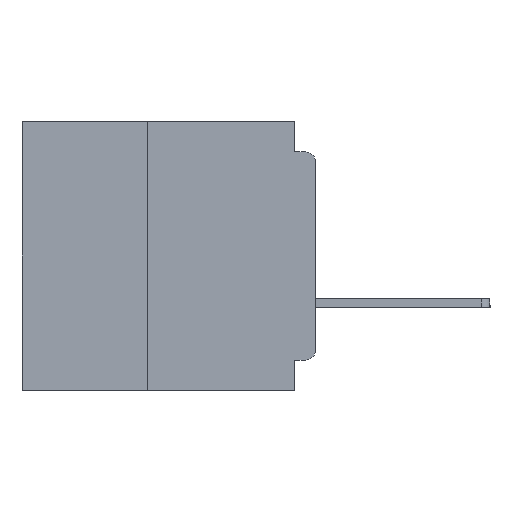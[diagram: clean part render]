
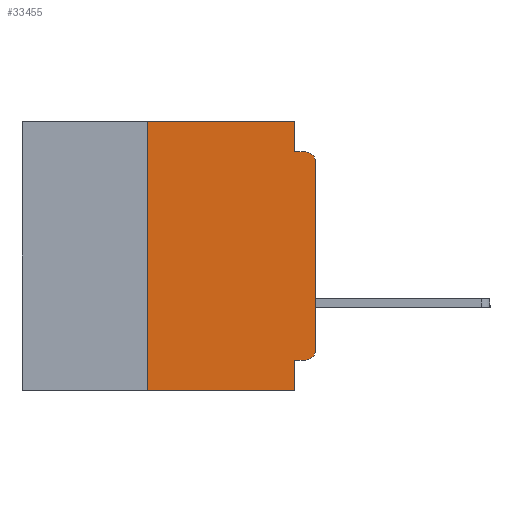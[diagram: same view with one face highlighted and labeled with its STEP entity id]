
A CAD part, left-side view. The second image highlights one B-rep face of the part: STEP entity #33455.
In plain terms, the highlighted planar face has unit normal (-1, 0, 0).
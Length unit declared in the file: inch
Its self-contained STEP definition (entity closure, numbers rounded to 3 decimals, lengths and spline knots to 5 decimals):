
#30 = LINE ( 'NONE', #48279, #38272 ) ;
#171 = EDGE_CURVE ( 'NONE', #45101, #15262, #49814, .T. ) ;
#313 = ORIENTED_EDGE ( 'NONE', *, *, #45970, .F. ) ;
#551 = EDGE_CURVE ( 'NONE', #40416, #3719, #44306, .T. ) ;
#1659 = VECTOR ( 'NONE', #46915, 39.37008 ) ;
#2421 = CARTESIAN_POINT ( 'NONE',  ( 0., 0.031, 0. ) ) ;
#3719 = VERTEX_POINT ( 'NONE', #20917 ) ;
#3792 = LINE ( 'NONE', #22069, #23564 ) ;
#4035 = ORIENTED_EDGE ( 'NONE', *, *, #551, .F. ) ;
#8133 = EDGE_CURVE ( 'NONE', #45101, #36165, #47011, .T. ) ;
#9137 = DIRECTION ( 'NONE',  ( 0., 0., -1. ) ) ;
#9287 = DIRECTION ( 'NONE',  ( 0., 0., 1. ) ) ;
#9511 = DIRECTION ( 'NONE',  ( 0., 0., 1. ) ) ;
#9657 = CARTESIAN_POINT ( 'NONE',  ( 0., 0.015, -0.34 ) ) ;
#10088 = VERTEX_POINT ( 'NONE', #45412 ) ;
#10184 = ORIENTED_EDGE ( 'NONE', *, *, #13428, .F. ) ;
#11434 = AXIS2_PLACEMENT_3D ( 'NONE', #20685, #48061, #24645 ) ;
#12172 = LINE ( 'NONE', #31227, #1659 ) ;
#12761 = LINE ( 'NONE', #40751, #50782 ) ;
#12777 = FACE_OUTER_BOUND ( 'NONE', #46344, .T. ) ;
#12969 = VECTOR ( 'NONE', #26232, 39.37008 ) ;
#13257 = ORIENTED_EDGE ( 'NONE', *, *, #41112, .T. ) ;
#13428 = EDGE_CURVE ( 'NONE', #44239, #15635, #27685, .T. ) ;
#13634 = DIRECTION ( 'NONE',  ( 0., 0., -1. ) ) ;
#14319 = CARTESIAN_POINT ( 'NONE',  ( 0., 0.25, 0. ) ) ;
#15262 = VERTEX_POINT ( 'NONE', #15535 ) ;
#15535 = CARTESIAN_POINT ( 'NONE',  ( 0., 0.031, -0.4 ) ) ;
#15635 = VERTEX_POINT ( 'NONE', #22401 ) ;
#15716 = VECTOR ( 'NONE', #9511, 39.37008 ) ;
#15987 = VECTOR ( 'NONE', #24938, 39.37008 ) ;
#16967 = ORIENTED_EDGE ( 'NONE', *, *, #19109, .F. ) ;
#17752 = DIRECTION ( 'NONE',  ( 0., -1., 0. ) ) ;
#18827 = CARTESIAN_POINT ( 'NONE',  ( 0., 0., -0.34 ) ) ;
#19109 = EDGE_CURVE ( 'NONE', #15635, #42695, #3792, .T. ) ;
#19437 = CARTESIAN_POINT ( 'NONE',  ( 0., 0.25, -0.4 ) ) ;
#19502 = CARTESIAN_POINT ( 'NONE',  ( 0., 0.437, 0. ) ) ;
#19772 = CIRCLE ( 'NONE', #11434, 0.015 ) ;
#20685 = CARTESIAN_POINT ( 'NONE',  ( 0., 0.015, -0.06 ) ) ;
#20917 = CARTESIAN_POINT ( 'NONE',  ( 0., 0.031, -0.355 ) ) ;
#20986 = CARTESIAN_POINT ( 'NONE',  ( 0., 0.031, 0. ) ) ;
#20989 = CARTESIAN_POINT ( 'NONE',  ( 0., 0.437, -0.4 ) ) ;
#22069 = CARTESIAN_POINT ( 'NONE',  ( 0., 0., -0.045 ) ) ;
#22242 = DIRECTION ( 'NONE',  ( 0., -1., 0. ) ) ;
#22401 = CARTESIAN_POINT ( 'NONE',  ( 0., 0.031, -0.045 ) ) ;
#22969 = CARTESIAN_POINT ( 'NONE',  ( 0., 0., -0.355 ) ) ;
#23477 = DIRECTION ( 'NONE',  ( 0., 0., -1. ) ) ;
#23564 = VECTOR ( 'NONE', #22242, 39.37008 ) ;
#24240 = CIRCLE ( 'NONE', #46910, 0.015 ) ;
#24417 = ORIENTED_EDGE ( 'NONE', *, *, #8133, .F. ) ;
#24645 = DIRECTION ( 'NONE',  ( 0., 0., -1. ) ) ;
#24938 = DIRECTION ( 'NONE',  ( 0., 0., -1. ) ) ;
#26232 = DIRECTION ( 'NONE',  ( 0., 1., 0. ) ) ;
#27685 = LINE ( 'NONE', #20986, #15987 ) ;
#28710 = ORIENTED_EDGE ( 'NONE', *, *, #30641, .T. ) ;
#29152 = CARTESIAN_POINT ( 'NONE',  ( 0., 0.25, -0.4 ) ) ;
#30289 = VECTOR ( 'NONE', #17752, 39.37008 ) ;
#30641 = EDGE_CURVE ( 'NONE', #40416, #44302, #24240, .T. ) ;
#31167 = ORIENTED_EDGE ( 'NONE', *, *, #42493, .F. ) ;
#31227 = CARTESIAN_POINT ( 'NONE',  ( 0., 0.437, 0. ) ) ;
#33455 = ADVANCED_FACE ( 'NONE', ( #12777 ), #42973, .F. ) ;
#35858 = CARTESIAN_POINT ( 'NONE',  ( 0., 0.015, -0.355 ) ) ;
#36165 = VERTEX_POINT ( 'NONE', #14319 ) ;
#37200 = DIRECTION ( 'NONE',  ( -1., 0., 0. ) ) ;
#38272 = VECTOR ( 'NONE', #9137, 39.37008 ) ;
#39702 = ORIENTED_EDGE ( 'NONE', *, *, #42759, .T. ) ;
#40416 = VERTEX_POINT ( 'NONE', #35858 ) ;
#40751 = CARTESIAN_POINT ( 'NONE',  ( 0., 0., 0. ) ) ;
#41112 = EDGE_CURVE ( 'NONE', #10088, #42695, #19772, .T. ) ;
#42493 = EDGE_CURVE ( 'NONE', #36165, #44239, #12172, .T. ) ;
#42695 = VERTEX_POINT ( 'NONE', #44331 ) ;
#42759 = EDGE_CURVE ( 'NONE', #44302, #10088, #12761, .T. ) ;
#42973 = PLANE ( 'NONE',  #45727 ) ;
#44239 = VERTEX_POINT ( 'NONE', #2421 ) ;
#44302 = VERTEX_POINT ( 'NONE', #18827 ) ;
#44306 = LINE ( 'NONE', #22969, #12969 ) ;
#44331 = CARTESIAN_POINT ( 'NONE',  ( 0., 0.015, -0.045 ) ) ;
#45101 = VERTEX_POINT ( 'NONE', #19437 ) ;
#45412 = CARTESIAN_POINT ( 'NONE',  ( 0., 0., -0.06 ) ) ;
#45727 = AXIS2_PLACEMENT_3D ( 'NONE', #19502, #46901, #23477 ) ;
#45970 = EDGE_CURVE ( 'NONE', #3719, #15262, #30, .T. ) ;
#46344 = EDGE_LOOP ( 'NONE', ( #39702, #13257, #16967, #10184, #31167, #24417, #46434, #313, #4035, #28710 ) ) ;
#46434 = ORIENTED_EDGE ( 'NONE', *, *, #171, .T. ) ;
#46901 = DIRECTION ( 'NONE',  ( 1., 0., 0. ) ) ;
#46910 = AXIS2_PLACEMENT_3D ( 'NONE', #9657, #37200, #13634 ) ;
#46915 = DIRECTION ( 'NONE',  ( 0., -1., 0. ) ) ;
#47011 = LINE ( 'NONE', #29152, #15716 ) ;
#48061 = DIRECTION ( 'NONE',  ( -1., 0., 0. ) ) ;
#48279 = CARTESIAN_POINT ( 'NONE',  ( 0., 0.031, -0.4 ) ) ;
#49814 = LINE ( 'NONE', #20989, #30289 ) ;
#50782 = VECTOR ( 'NONE', #9287, 39.37008 ) ;
